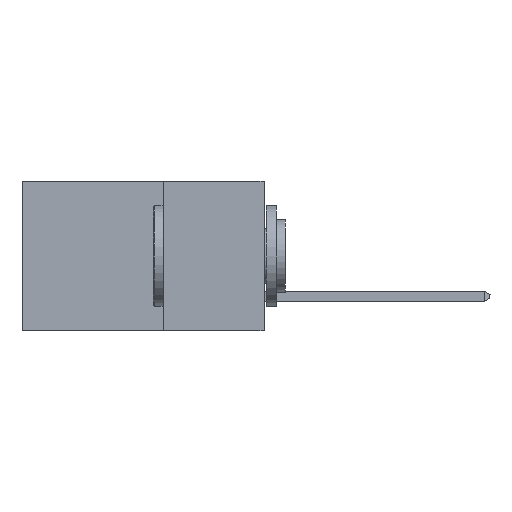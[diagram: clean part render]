
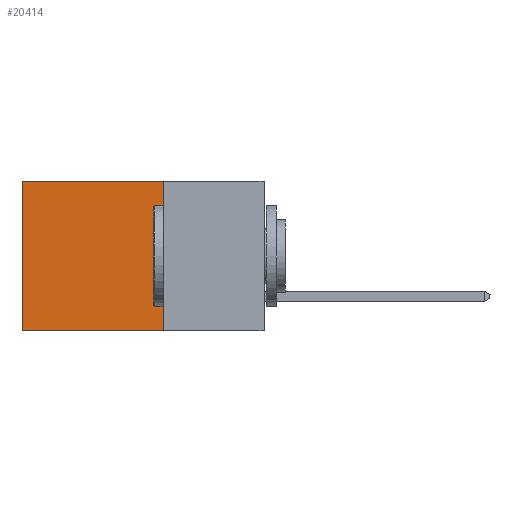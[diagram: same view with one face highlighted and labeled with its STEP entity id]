
A CAD part, left-side view. The second image highlights one B-rep face of the part: STEP entity #20414.
In plain terms, the highlighted planar face has unit normal (-1, 0, 0).
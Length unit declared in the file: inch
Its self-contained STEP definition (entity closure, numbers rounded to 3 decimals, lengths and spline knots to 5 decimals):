
#209 = VERTEX_POINT ( 'NONE', #13706 ) ;
#1149 = DIRECTION ( 'NONE',  ( 0., 0., -1. ) ) ;
#1501 = EDGE_CURVE ( 'NONE', #209, #17872, #2483, .T. ) ;
#2142 = LINE ( 'NONE', #14836, #9154 ) ;
#2193 = ORIENTED_EDGE ( 'NONE', *, *, #12528, .F. ) ;
#2444 = ORIENTED_EDGE ( 'NONE', *, *, #11008, .T. ) ;
#2483 = LINE ( 'NONE', #7359, #13254 ) ;
#2865 = CARTESIAN_POINT ( 'NONE',  ( 0.2615, 0.25, -0.37 ) ) ;
#3796 = DIRECTION ( 'NONE',  ( 0., 0., -1. ) ) ;
#3928 = VECTOR ( 'NONE', #14099, 39.37008 ) ;
#3935 = DIRECTION ( 'NONE',  ( 0., 1., 0. ) ) ;
#4174 = CARTESIAN_POINT ( 'NONE',  ( 0.2615, 0.25, -0.37 ) ) ;
#4672 = DIRECTION ( 'NONE',  ( 1., 0., 0. ) ) ;
#5865 = LINE ( 'NONE', #2865, #3928 ) ;
#6128 = CARTESIAN_POINT ( 'NONE',  ( 0.2615, 0.25, -0.37 ) ) ;
#6531 = DIRECTION ( 'NONE',  ( 0., 0., -1. ) ) ;
#6596 = VECTOR ( 'NONE', #1149, 39.37008 ) ;
#7070 = AXIS2_PLACEMENT_3D ( 'NONE', #6128, #4672, #6531 ) ;
#7359 = CARTESIAN_POINT ( 'NONE',  ( 0.2615, 0.25, 0. ) ) ;
#7797 = PLANE ( 'NONE',  #7070 ) ;
#7992 = FACE_OUTER_BOUND ( 'NONE', #18064, .T. ) ;
#8892 = CARTESIAN_POINT ( 'NONE',  ( 0.2615, 0.25, -0.37 ) ) ;
#9154 = VECTOR ( 'NONE', #3796, 39.37008 ) ;
#10805 = VERTEX_POINT ( 'NONE', #10974 ) ;
#10974 = CARTESIAN_POINT ( 'NONE',  ( 0.2615, 0.6, -0.37 ) ) ;
#11008 = EDGE_CURVE ( 'NONE', #17872, #10805, #2142, .T. ) ;
#12528 = EDGE_CURVE ( 'NONE', #209, #14596, #15413, .T. ) ;
#13254 = VECTOR ( 'NONE', #3935, 39.37008 ) ;
#13433 = EDGE_CURVE ( 'NONE', #14596, #10805, #5865, .T. ) ;
#13706 = CARTESIAN_POINT ( 'NONE',  ( 0.2615, 0.25, 0. ) ) ;
#14099 = DIRECTION ( 'NONE',  ( 0., 1., 0. ) ) ;
#14420 = ORIENTED_EDGE ( 'NONE', *, *, #1501, .T. ) ;
#14596 = VERTEX_POINT ( 'NONE', #8892 ) ;
#14836 = CARTESIAN_POINT ( 'NONE',  ( 0.2615, 0.6, -0.37 ) ) ;
#14945 = ORIENTED_EDGE ( 'NONE', *, *, #13433, .F. ) ;
#15413 = LINE ( 'NONE', #4174, #6596 ) ;
#16222 = CARTESIAN_POINT ( 'NONE',  ( 0.2615, 0.6, 0. ) ) ;
#17872 = VERTEX_POINT ( 'NONE', #16222 ) ;
#18064 = EDGE_LOOP ( 'NONE', ( #2444, #14945, #2193, #14420 ) ) ;
#20414 = ADVANCED_FACE ( 'NONE', ( #7992 ), #7797, .F. ) ;
